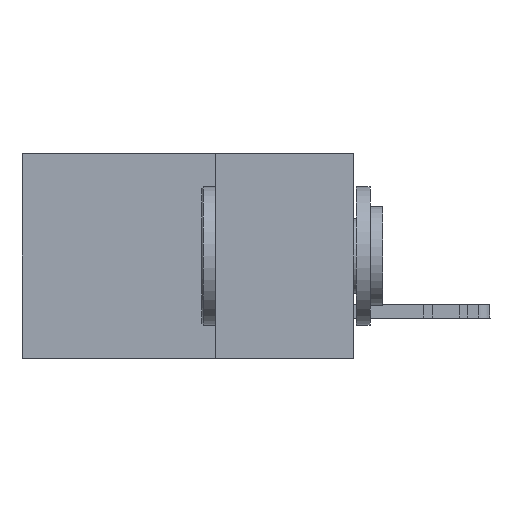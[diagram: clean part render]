
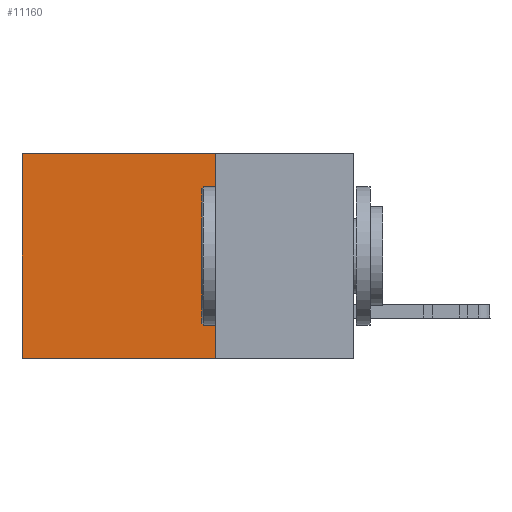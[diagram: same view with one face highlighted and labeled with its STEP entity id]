
A CAD part, left-side view. The second image highlights one B-rep face of the part: STEP entity #11160.
In plain terms, the highlighted planar face has unit normal (-1, 0, 0).
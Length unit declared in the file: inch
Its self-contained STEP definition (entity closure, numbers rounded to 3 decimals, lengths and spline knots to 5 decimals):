
#1663 = VECTOR ( 'NONE', #7090, 39.37008 ) ;
#4093 = VERTEX_POINT ( 'NONE', #34234 ) ;
#5496 = EDGE_CURVE ( 'NONE', #4093, #9613, #10713, .T. ) ;
#5629 = LINE ( 'NONE', #13062, #28586 ) ;
#5657 = DIRECTION ( 'NONE',  ( 1., 0., 0. ) ) ;
#6879 = CARTESIAN_POINT ( 'NONE',  ( 0.2875, 0.25, 0. ) ) ;
#7090 = DIRECTION ( 'NONE',  ( 0., 1., 0. ) ) ;
#9613 = VERTEX_POINT ( 'NONE', #19913 ) ;
#10606 = VECTOR ( 'NONE', #31165, 39.37008 ) ;
#10713 = LINE ( 'NONE', #21536, #43295 ) ;
#11160 = ADVANCED_FACE ( 'NONE', ( #36332 ), #36555, .F. ) ;
#12649 = DIRECTION ( 'NONE',  ( 0., 0., -1. ) ) ;
#13062 = CARTESIAN_POINT ( 'NONE',  ( 0.2875, 0.25, -0.37 ) ) ;
#15787 = DIRECTION ( 'NONE',  ( 0., 1., 0. ) ) ;
#17404 = LINE ( 'NONE', #41080, #10606 ) ;
#18174 = ORIENTED_EDGE ( 'NONE', *, *, #40534, .T. ) ;
#19913 = CARTESIAN_POINT ( 'NONE',  ( 0.2875, 0.6, -0.37 ) ) ;
#20783 = EDGE_CURVE ( 'NONE', #25573, #9613, #5629, .T. ) ;
#21528 = LINE ( 'NONE', #41808, #1663 ) ;
#21536 = CARTESIAN_POINT ( 'NONE',  ( 0.2875, 0.6, 0. ) ) ;
#22074 = CARTESIAN_POINT ( 'NONE',  ( 0.2875, 0.25, -0.37 ) ) ;
#25573 = VERTEX_POINT ( 'NONE', #22074 ) ;
#27697 = ORIENTED_EDGE ( 'NONE', *, *, #31276, .F. ) ;
#27869 = ORIENTED_EDGE ( 'NONE', *, *, #5496, .T. ) ;
#28586 = VECTOR ( 'NONE', #15787, 39.37008 ) ;
#28819 = VERTEX_POINT ( 'NONE', #6879 ) ;
#29159 = AXIS2_PLACEMENT_3D ( 'NONE', #43317, #5657, #12649 ) ;
#31165 = DIRECTION ( 'NONE',  ( 0., 0., -1. ) ) ;
#31276 = EDGE_CURVE ( 'NONE', #28819, #25573, #17404, .T. ) ;
#31446 = DIRECTION ( 'NONE',  ( 0., 0., -1. ) ) ;
#33754 = EDGE_LOOP ( 'NONE', ( #27869, #43937, #27697, #18174 ) ) ;
#34234 = CARTESIAN_POINT ( 'NONE',  ( 0.2875, 0.6, 0. ) ) ;
#36332 = FACE_OUTER_BOUND ( 'NONE', #33754, .T. ) ;
#36555 = PLANE ( 'NONE',  #29159 ) ;
#40534 = EDGE_CURVE ( 'NONE', #28819, #4093, #21528, .T. ) ;
#41080 = CARTESIAN_POINT ( 'NONE',  ( 0.2875, 0.25, 0. ) ) ;
#41808 = CARTESIAN_POINT ( 'NONE',  ( 0.2875, 0.25, 0. ) ) ;
#43295 = VECTOR ( 'NONE', #31446, 39.37008 ) ;
#43317 = CARTESIAN_POINT ( 'NONE',  ( 0.2875, 0.25, 0. ) ) ;
#43937 = ORIENTED_EDGE ( 'NONE', *, *, #20783, .F. ) ;
